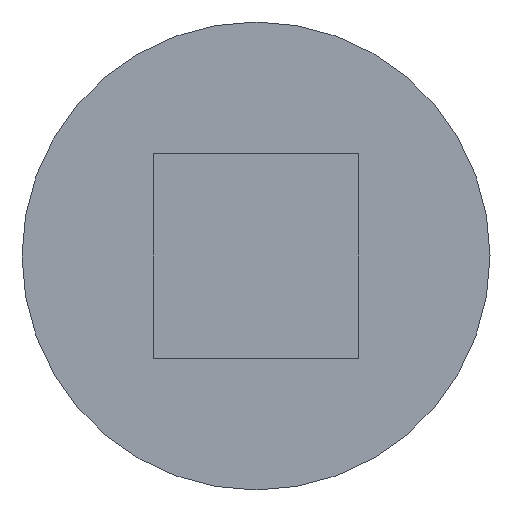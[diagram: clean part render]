
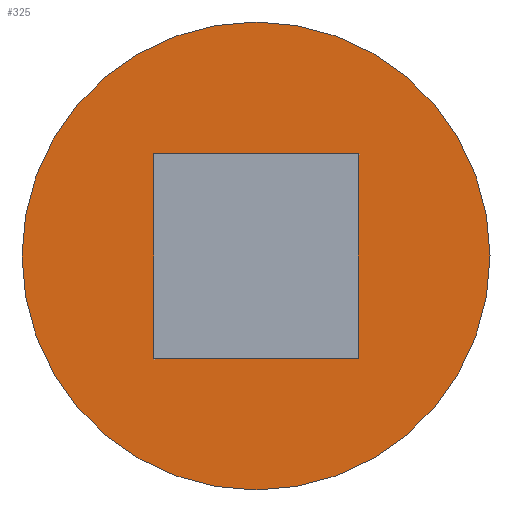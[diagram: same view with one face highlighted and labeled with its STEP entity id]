
A CAD part, left-side view. The second image highlights one B-rep face of the part: STEP entity #325.
In plain terms, the highlighted planar face has unit normal (-1, 0, 0).
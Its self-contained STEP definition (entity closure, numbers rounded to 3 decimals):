
#20=FACE_BOUND('',#64,.T.);
#40=FACE_OUTER_BOUND('',#63,.T.);
#63=EDGE_LOOP('',(#267));
#64=EDGE_LOOP('',(#268,#269,#270,#271));
#78=CIRCLE('',#358,12.7);
#104=LINE('',#521,#134);
#108=LINE('',#529,#138);
#111=LINE('',#535,#141);
#114=LINE('',#540,#144);
#134=VECTOR('',#411,10.);
#138=VECTOR('',#417,10.);
#141=VECTOR('',#422,10.);
#144=VECTOR('',#427,10.);
#165=VERTEX_POINT('',#519);
#166=VERTEX_POINT('',#520);
#169=VERTEX_POINT('',#528);
#171=VERTEX_POINT('',#534);
#174=VERTEX_POINT('',#548);
#196=EDGE_CURVE('',#165,#166,#104,.T.);
#200=EDGE_CURVE('',#166,#169,#108,.T.);
#203=EDGE_CURVE('',#169,#171,#111,.T.);
#206=EDGE_CURVE('',#171,#165,#114,.T.);
#210=EDGE_CURVE('',#174,#174,#78,.T.);
#267=ORIENTED_EDGE('',*,*,#210,.T.);
#268=ORIENTED_EDGE('',*,*,#196,.T.);
#269=ORIENTED_EDGE('',*,*,#200,.T.);
#270=ORIENTED_EDGE('',*,*,#203,.T.);
#271=ORIENTED_EDGE('',*,*,#206,.T.);
#313=PLANE('',#359);
#325=ADVANCED_FACE('',(#40,#20),#313,.T.);
#358=AXIS2_PLACEMENT_3D('',#549,#439,#440);
#359=AXIS2_PLACEMENT_3D('',#550,#441,#442);
#411=DIRECTION('',(0.,-1.,0.));
#417=DIRECTION('',(0.,0.,-1.));
#422=DIRECTION('',(0.,1.,0.));
#427=DIRECTION('',(0.,0.,1.));
#439=DIRECTION('center_axis',(-1.,0.,0.));
#440=DIRECTION('ref_axis',(0.,0.,-1.));
#441=DIRECTION('center_axis',(-1.,0.,0.));
#442=DIRECTION('ref_axis',(0.,0.,1.));
#519=CARTESIAN_POINT('',(-12.7,5.556,5.556));
#520=CARTESIAN_POINT('',(-12.7,-5.556,5.556));
#521=CARTESIAN_POINT('',(-12.7,-2.778,5.556));
#528=CARTESIAN_POINT('',(-12.7,-5.556,-5.556));
#529=CARTESIAN_POINT('',(-12.7,-5.556,-2.778));
#534=CARTESIAN_POINT('',(-12.7,5.556,-5.556));
#535=CARTESIAN_POINT('',(-12.7,2.778,-5.556));
#540=CARTESIAN_POINT('',(-12.7,5.556,2.778));
#548=CARTESIAN_POINT('',(-12.7,0.,12.7));
#549=CARTESIAN_POINT('Origin',(-12.7,0.,0.));
#550=CARTESIAN_POINT('Origin',(-12.7,0.,0.));
